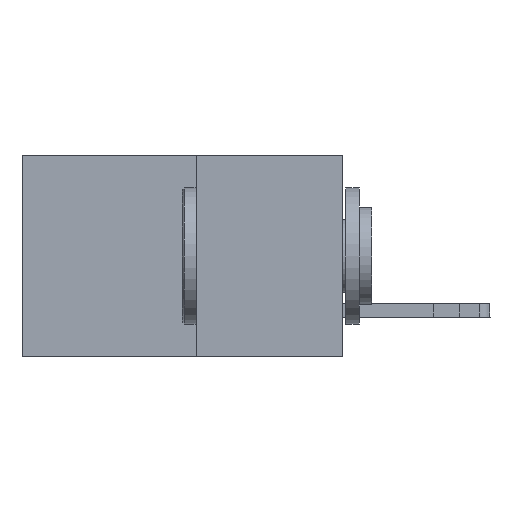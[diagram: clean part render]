
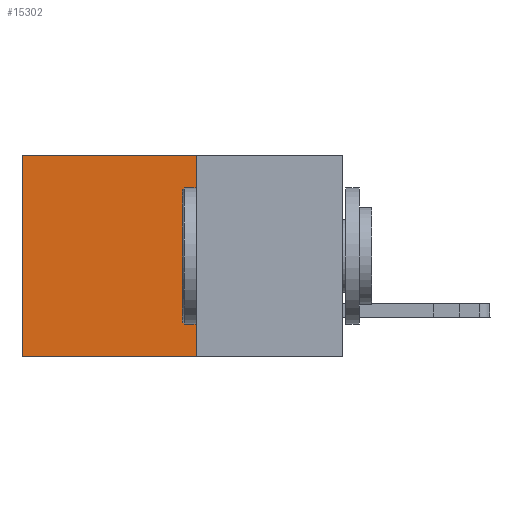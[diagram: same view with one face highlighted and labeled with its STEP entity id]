
A CAD part, left-side view. The second image highlights one B-rep face of the part: STEP entity #15302.
In plain terms, the highlighted planar face has unit normal (-1, 0, 0).
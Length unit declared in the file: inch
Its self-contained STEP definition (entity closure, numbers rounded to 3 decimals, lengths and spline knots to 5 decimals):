
#149 = VECTOR ( 'NONE', #7399, 39.37008 ) ;
#151 = EDGE_LOOP ( 'NONE', ( #11023, #15859, #12173, #13547 ) ) ;
#1407 = VECTOR ( 'NONE', #12468, 39.37008 ) ;
#2068 = CARTESIAN_POINT ( 'NONE',  ( 0.277, 0.27, -0.37 ) ) ;
#2279 = PLANE ( 'NONE',  #11458 ) ;
#2769 = EDGE_CURVE ( 'NONE', #11370, #3563, #6255, .T. ) ;
#3563 = VERTEX_POINT ( 'NONE', #2068 ) ;
#3652 = DIRECTION ( 'NONE',  ( 1., 0., 0. ) ) ;
#4070 = VECTOR ( 'NONE', #15897, 39.37008 ) ;
#5069 = LINE ( 'NONE', #12487, #1407 ) ;
#5221 = EDGE_CURVE ( 'NONE', #3563, #12001, #5069, .T. ) ;
#6195 = CARTESIAN_POINT ( 'NONE',  ( 0.277, 0.59, -0.37 ) ) ;
#6255 = LINE ( 'NONE', #12707, #17347 ) ;
#6790 = LINE ( 'NONE', #6195, #4070 ) ;
#7399 = DIRECTION ( 'NONE',  ( 0., 1., 0. ) ) ;
#7511 = FACE_OUTER_BOUND ( 'NONE', #151, .T. ) ;
#8299 = EDGE_CURVE ( 'NONE', #12107, #12001, #6790, .T. ) ;
#9591 = CARTESIAN_POINT ( 'NONE',  ( 0.277, 0.59, -0.37 ) ) ;
#10513 = CARTESIAN_POINT ( 'NONE',  ( 0.277, 0.27, -0.37 ) ) ;
#11023 = ORIENTED_EDGE ( 'NONE', *, *, #8299, .T. ) ;
#11178 = LINE ( 'NONE', #15666, #149 ) ;
#11370 = VERTEX_POINT ( 'NONE', #16494 ) ;
#11458 = AXIS2_PLACEMENT_3D ( 'NONE', #10513, #3652, #13373 ) ;
#12001 = VERTEX_POINT ( 'NONE', #9591 ) ;
#12107 = VERTEX_POINT ( 'NONE', #15423 ) ;
#12173 = ORIENTED_EDGE ( 'NONE', *, *, #2769, .F. ) ;
#12468 = DIRECTION ( 'NONE',  ( 0., 1., 0. ) ) ;
#12487 = CARTESIAN_POINT ( 'NONE',  ( 0.277, 0.27, -0.37 ) ) ;
#12707 = CARTESIAN_POINT ( 'NONE',  ( 0.277, 0.27, -0.37 ) ) ;
#13373 = DIRECTION ( 'NONE',  ( 0., 0., -1. ) ) ;
#13547 = ORIENTED_EDGE ( 'NONE', *, *, #15087, .T. ) ;
#15087 = EDGE_CURVE ( 'NONE', #11370, #12107, #11178, .T. ) ;
#15302 = ADVANCED_FACE ( 'NONE', ( #7511 ), #2279, .F. ) ;
#15423 = CARTESIAN_POINT ( 'NONE',  ( 0.277, 0.59, 0. ) ) ;
#15666 = CARTESIAN_POINT ( 'NONE',  ( 0.277, 0.27, 0. ) ) ;
#15859 = ORIENTED_EDGE ( 'NONE', *, *, #5221, .F. ) ;
#15897 = DIRECTION ( 'NONE',  ( 0., 0., -1. ) ) ;
#16288 = DIRECTION ( 'NONE',  ( 0., 0., -1. ) ) ;
#16494 = CARTESIAN_POINT ( 'NONE',  ( 0.277, 0.27, 0. ) ) ;
#17347 = VECTOR ( 'NONE', #16288, 39.37008 ) ;
